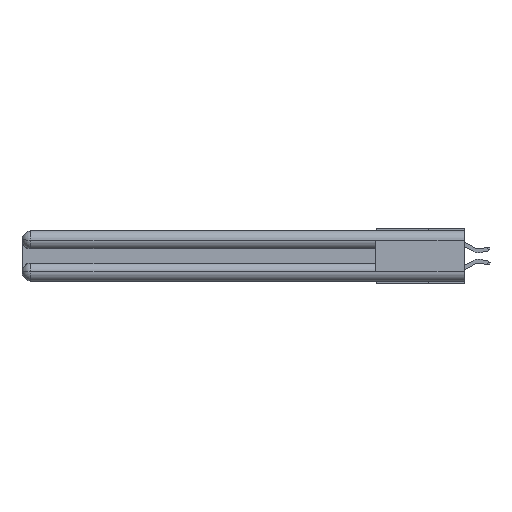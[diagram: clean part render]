
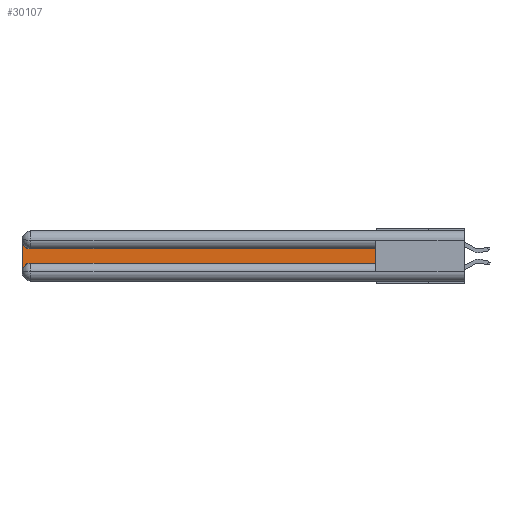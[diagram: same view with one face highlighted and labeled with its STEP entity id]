
A CAD part, left-side view. The second image highlights one B-rep face of the part: STEP entity #30107.
In plain terms, the highlighted planar face has unit normal (-1, 0, 0).
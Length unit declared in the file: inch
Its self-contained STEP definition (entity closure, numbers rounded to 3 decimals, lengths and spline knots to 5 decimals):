
#266 = CARTESIAN_POINT ( 'NONE',  ( 0.075, 3., -0.0625 ) ) ;
#915 = DIRECTION ( 'NONE',  ( 0., 0., 1. ) ) ;
#1731 = VERTEX_POINT ( 'NONE', #20674 ) ;
#2315 = VECTOR ( 'NONE', #18044, 39.37008 ) ;
#5111 = VERTEX_POINT ( 'NONE', #26023 ) ;
#5369 = ORIENTED_EDGE ( 'NONE', *, *, #28774, .T. ) ;
#5410 = EDGE_CURVE ( 'NONE', #21503, #11558, #30609, .T. ) ;
#6746 = EDGE_CURVE ( 'NONE', #30482, #11779, #33622, .T. ) ;
#8669 = ORIENTED_EDGE ( 'NONE', *, *, #18315, .T. ) ;
#9220 = AXIS2_PLACEMENT_3D ( 'NONE', #34601, #23478, #20562 ) ;
#9910 = DIRECTION ( 'NONE',  ( 0., 1., 0. ) ) ;
#10109 = VECTOR ( 'NONE', #33123, 39.37008 ) ;
#10340 = DIRECTION ( 'NONE',  ( 1., 0., 0. ) ) ;
#11558 = VERTEX_POINT ( 'NONE', #25922 ) ;
#11779 = VERTEX_POINT ( 'NONE', #12834 ) ;
#12722 = ORIENTED_EDGE ( 'NONE', *, *, #30347, .T. ) ;
#12834 = CARTESIAN_POINT ( 'NONE',  ( 0.075, 0.6, -0.1225 ) ) ;
#13347 = CARTESIAN_POINT ( 'NONE',  ( 0.075, 0.6, -0.2175 ) ) ;
#15366 = CARTESIAN_POINT ( 'NONE',  ( 0.075, 3., -0.2175 ) ) ;
#15488 = DIRECTION ( 'NONE',  ( 0., 0., -1. ) ) ;
#17319 = CIRCLE ( 'NONE', #19063, 0.06 ) ;
#18044 = DIRECTION ( 'NONE',  ( 0., 0., -1. ) ) ;
#18315 = EDGE_CURVE ( 'NONE', #1731, #21503, #20306, .T. ) ;
#19063 = AXIS2_PLACEMENT_3D ( 'NONE', #35111, #10340, #21432 ) ;
#20306 = CIRCLE ( 'NONE', #34709, 0.06 ) ;
#20562 = DIRECTION ( 'NONE',  ( 0., 0., -1. ) ) ;
#20674 = CARTESIAN_POINT ( 'NONE',  ( 0.075, 2.94, -0.1225 ) ) ;
#21432 = DIRECTION ( 'NONE',  ( 0., 0., -1. ) ) ;
#21503 = VERTEX_POINT ( 'NONE', #266 ) ;
#21609 = EDGE_LOOP ( 'NONE', ( #5369, #8669, #31386, #26151, #12722, #33689 ) ) ;
#22087 = CARTESIAN_POINT ( 'NONE',  ( 0.075, 0.6, -0.2175 ) ) ;
#22479 = EDGE_CURVE ( 'NONE', #11558, #5111, #17319, .T. ) ;
#23222 = PLANE ( 'NONE',  #9220 ) ;
#23437 = CARTESIAN_POINT ( 'NONE',  ( 0.075, 0.6, -0.1225 ) ) ;
#23478 = DIRECTION ( 'NONE',  ( 1., 0., 0. ) ) ;
#23708 = LINE ( 'NONE', #23437, #29828 ) ;
#23934 = CARTESIAN_POINT ( 'NONE',  ( 0.075, 2.94, -0.0625 ) ) ;
#25922 = CARTESIAN_POINT ( 'NONE',  ( 0.075, 3., -0.2775 ) ) ;
#26023 = CARTESIAN_POINT ( 'NONE',  ( 0.075, 2.94, -0.2175 ) ) ;
#26151 = ORIENTED_EDGE ( 'NONE', *, *, #22479, .T. ) ;
#26838 = DIRECTION ( 'NONE',  ( 1., 0., 0. ) ) ;
#28419 = FACE_OUTER_BOUND ( 'NONE', #21609, .T. ) ;
#28774 = EDGE_CURVE ( 'NONE', #11779, #1731, #23708, .T. ) ;
#29828 = VECTOR ( 'NONE', #9910, 39.37008 ) ;
#30107 = ADVANCED_FACE ( 'NONE', ( #28419 ), #23222, .F. ) ;
#30347 = EDGE_CURVE ( 'NONE', #5111, #30482, #30616, .T. ) ;
#30482 = VERTEX_POINT ( 'NONE', #22087 ) ;
#30609 = LINE ( 'NONE', #15366, #2315 ) ;
#30616 = LINE ( 'NONE', #13347, #10109 ) ;
#31386 = ORIENTED_EDGE ( 'NONE', *, *, #5410, .T. ) ;
#31501 = CARTESIAN_POINT ( 'NONE',  ( 0.075, 0.6, -0.2175 ) ) ;
#33123 = DIRECTION ( 'NONE',  ( 0., -1., 0. ) ) ;
#33622 = LINE ( 'NONE', #31501, #35380 ) ;
#33689 = ORIENTED_EDGE ( 'NONE', *, *, #6746, .T. ) ;
#34601 = CARTESIAN_POINT ( 'NONE',  ( 0.075, 3., -0.1225 ) ) ;
#34709 = AXIS2_PLACEMENT_3D ( 'NONE', #23934, #26838, #15488 ) ;
#35111 = CARTESIAN_POINT ( 'NONE',  ( 0.075, 2.94, -0.2775 ) ) ;
#35380 = VECTOR ( 'NONE', #915, 39.37008 ) ;
